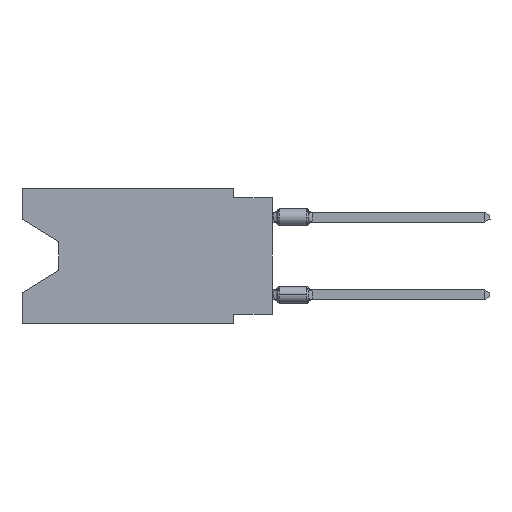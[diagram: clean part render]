
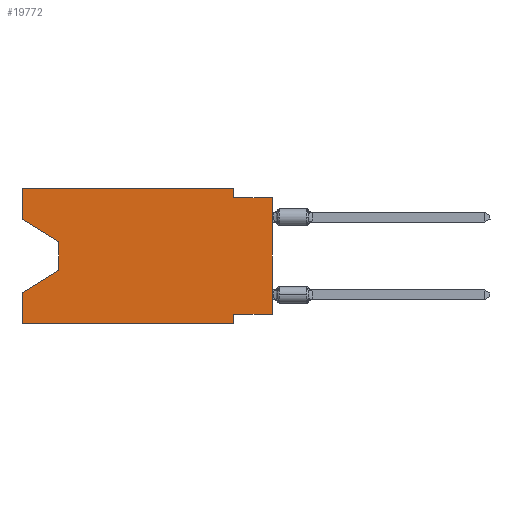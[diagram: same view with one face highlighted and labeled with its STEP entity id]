
A CAD part, left-side view. The second image highlights one B-rep face of the part: STEP entity #19772.
In plain terms, the highlighted planar face has unit normal (-1, 0, 0).
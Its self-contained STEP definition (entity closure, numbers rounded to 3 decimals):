
#196 = CARTESIAN_POINT ( 'NONE',  ( 0., 2.54, -8.89 ) ) ;
#376 = EDGE_CURVE ( 'NONE', #31185, #6942, #43615, .T. ) ;
#868 = EDGE_CURVE ( 'NONE', #23839, #10003, #36662, .T. ) ;
#2128 = VECTOR ( 'NONE', #16465, 1000. ) ;
#2604 = CARTESIAN_POINT ( 'NONE',  ( 0., 16.383, 0. ) ) ;
#3965 = LINE ( 'NONE', #24300, #13860 ) ;
#4038 = CARTESIAN_POINT ( 'NONE',  ( 0., 2.54, 0. ) ) ;
#4153 = LINE ( 'NONE', #196, #47601 ) ;
#5309 = ORIENTED_EDGE ( 'NONE', *, *, #12894, .F. ) ;
#5824 = VERTEX_POINT ( 'NONE', #34287 ) ;
#6548 = ORIENTED_EDGE ( 'NONE', *, *, #6852, .F. ) ;
#6759 = DIRECTION ( 'NONE',  ( 0., -1., 0. ) ) ;
#6852 = EDGE_CURVE ( 'NONE', #6942, #11643, #43375, .T. ) ;
#6942 = VERTEX_POINT ( 'NONE', #4038 ) ;
#6943 = LINE ( 'NONE', #22799, #8994 ) ;
#7220 = CARTESIAN_POINT ( 'NONE',  ( 0., 2.54, 0. ) ) ;
#7282 = CARTESIAN_POINT ( 'NONE',  ( 0., 0., -8.255 ) ) ;
#7476 = DIRECTION ( 'NONE',  ( 0., -1., 0. ) ) ;
#7751 = DIRECTION ( 'NONE',  ( 0., 0., -1. ) ) ;
#8351 = ORIENTED_EDGE ( 'NONE', *, *, #22469, .T. ) ;
#8994 = VECTOR ( 'NONE', #22270, 1000. ) ;
#9380 = VERTEX_POINT ( 'NONE', #18475 ) ;
#10003 = VERTEX_POINT ( 'NONE', #39504 ) ;
#10662 = DIRECTION ( 'NONE',  ( 0., 0., -1. ) ) ;
#11643 = VERTEX_POINT ( 'NONE', #29091 ) ;
#12639 = LINE ( 'NONE', #24032, #48574 ) ;
#12894 = EDGE_CURVE ( 'NONE', #23839, #31185, #12639, .T. ) ;
#13431 = VERTEX_POINT ( 'NONE', #25521 ) ;
#13860 = VECTOR ( 'NONE', #28506, 1000. ) ;
#13978 = EDGE_CURVE ( 'NONE', #21627, #20810, #6943, .T. ) ;
#14074 = DIRECTION ( 'NONE',  ( 1., 0., 0. ) ) ;
#14176 = VERTEX_POINT ( 'NONE', #19610 ) ;
#16465 = DIRECTION ( 'NONE',  ( 0., 0.855, -0.519 ) ) ;
#17012 = EDGE_CURVE ( 'NONE', #10003, #17214, #49839, .T. ) ;
#17214 = VERTEX_POINT ( 'NONE', #40198 ) ;
#18475 = CARTESIAN_POINT ( 'NONE',  ( 0., 16.383, -6.852 ) ) ;
#18482 = ORIENTED_EDGE ( 'NONE', *, *, #45240, .F. ) ;
#18705 = DIRECTION ( 'NONE',  ( 0., 0., 1. ) ) ;
#19610 = CARTESIAN_POINT ( 'NONE',  ( 0., 2.54, -8.255 ) ) ;
#19745 = ORIENTED_EDGE ( 'NONE', *, *, #27910, .F. ) ;
#19765 = AXIS2_PLACEMENT_3D ( 'NONE', #41781, #14074, #34911 ) ;
#19772 = ADVANCED_FACE ( 'NONE', ( #34660 ), #42048, .F. ) ;
#20810 = VERTEX_POINT ( 'NONE', #41280 ) ;
#21374 = ORIENTED_EDGE ( 'NONE', *, *, #51829, .F. ) ;
#21627 = VERTEX_POINT ( 'NONE', #25570 ) ;
#22270 = DIRECTION ( 'NONE',  ( 0., -1., 0. ) ) ;
#22469 = EDGE_CURVE ( 'NONE', #17214, #9380, #49933, .T. ) ;
#22608 = CARTESIAN_POINT ( 'NONE',  ( 0., 0., -0.635 ) ) ;
#22799 = CARTESIAN_POINT ( 'NONE',  ( 0., 16.383, -8.89 ) ) ;
#22874 = LINE ( 'NONE', #22608, #38865 ) ;
#23386 = DIRECTION ( 'NONE',  ( 0., 1., 0. ) ) ;
#23839 = VERTEX_POINT ( 'NONE', #34662 ) ;
#24032 = CARTESIAN_POINT ( 'NONE',  ( 0., 16.383, 0. ) ) ;
#24300 = CARTESIAN_POINT ( 'NONE',  ( 0., 0., 0. ) ) ;
#24734 = DIRECTION ( 'NONE',  ( 0., 0., -1. ) ) ;
#25521 = CARTESIAN_POINT ( 'NONE',  ( 0., 0., -8.255 ) ) ;
#25570 = CARTESIAN_POINT ( 'NONE',  ( 0., 16.383, -8.89 ) ) ;
#27357 = LINE ( 'NONE', #7282, #40036 ) ;
#27910 = EDGE_CURVE ( 'NONE', #11643, #5824, #22874, .T. ) ;
#28506 = DIRECTION ( 'NONE',  ( 0., 0., 1. ) ) ;
#29091 = CARTESIAN_POINT ( 'NONE',  ( 0., 2.54, -0.635 ) ) ;
#29683 = EDGE_LOOP ( 'NONE', ( #45200, #32047, #8351, #18482, #49391, #30613, #21374, #50607, #19745, #6548, #42103, #5309 ) ) ;
#29851 = CARTESIAN_POINT ( 'NONE',  ( 0., 13.97, -5.385 ) ) ;
#30380 = VECTOR ( 'NONE', #7476, 1000. ) ;
#30613 = ORIENTED_EDGE ( 'NONE', *, *, #32143, .F. ) ;
#30734 = CARTESIAN_POINT ( 'NONE',  ( 0., 13.97, -3.505 ) ) ;
#31185 = VERTEX_POINT ( 'NONE', #43156 ) ;
#32047 = ORIENTED_EDGE ( 'NONE', *, *, #17012, .T. ) ;
#32122 = VECTOR ( 'NONE', #18705, 1000. ) ;
#32143 = EDGE_CURVE ( 'NONE', #14176, #20810, #4153, .T. ) ;
#32715 = DIRECTION ( 'NONE',  ( 0., -0.855, -0.519 ) ) ;
#33620 = VECTOR ( 'NONE', #7751, 1000. ) ;
#34287 = CARTESIAN_POINT ( 'NONE',  ( 0., 0., -0.635 ) ) ;
#34660 = FACE_OUTER_BOUND ( 'NONE', #29683, .T. ) ;
#34662 = CARTESIAN_POINT ( 'NONE',  ( 0., 16.383, -2.038 ) ) ;
#34911 = DIRECTION ( 'NONE',  ( 0., 0., -1. ) ) ;
#36662 = LINE ( 'NONE', #36920, #40562 ) ;
#36920 = CARTESIAN_POINT ( 'NONE',  ( 0., 16.383, -2.038 ) ) ;
#38865 = VECTOR ( 'NONE', #6759, 1000. ) ;
#39504 = CARTESIAN_POINT ( 'NONE',  ( 0., 13.97, -3.505 ) ) ;
#40036 = VECTOR ( 'NONE', #23386, 1000. ) ;
#40198 = CARTESIAN_POINT ( 'NONE',  ( 0., 13.97, -5.385 ) ) ;
#40562 = VECTOR ( 'NONE', #32715, 1000. ) ;
#41280 = CARTESIAN_POINT ( 'NONE',  ( 0., 2.54, -8.89 ) ) ;
#41781 = CARTESIAN_POINT ( 'NONE',  ( 0., 16.383, 0. ) ) ;
#42048 = PLANE ( 'NONE',  #19765 ) ;
#42103 = ORIENTED_EDGE ( 'NONE', *, *, #376, .F. ) ;
#42114 = VECTOR ( 'NONE', #10662, 1000. ) ;
#43156 = CARTESIAN_POINT ( 'NONE',  ( 0., 16.383, 0. ) ) ;
#43375 = LINE ( 'NONE', #7220, #33620 ) ;
#43615 = LINE ( 'NONE', #51809, #30380 ) ;
#45200 = ORIENTED_EDGE ( 'NONE', *, *, #868, .T. ) ;
#45240 = EDGE_CURVE ( 'NONE', #21627, #9380, #47211, .T. ) ;
#47211 = LINE ( 'NONE', #2604, #32122 ) ;
#47601 = VECTOR ( 'NONE', #24734, 1000. ) ;
#48565 = DIRECTION ( 'NONE',  ( 0., 0., 1. ) ) ;
#48574 = VECTOR ( 'NONE', #48565, 1000. ) ;
#49391 = ORIENTED_EDGE ( 'NONE', *, *, #13978, .T. ) ;
#49839 = LINE ( 'NONE', #30734, #42114 ) ;
#49933 = LINE ( 'NONE', #29851, #2128 ) ;
#50607 = ORIENTED_EDGE ( 'NONE', *, *, #51102, .T. ) ;
#51102 = EDGE_CURVE ( 'NONE', #13431, #5824, #3965, .T. ) ;
#51809 = CARTESIAN_POINT ( 'NONE',  ( 0., 16.383, 0. ) ) ;
#51829 = EDGE_CURVE ( 'NONE', #13431, #14176, #27357, .T. ) ;
